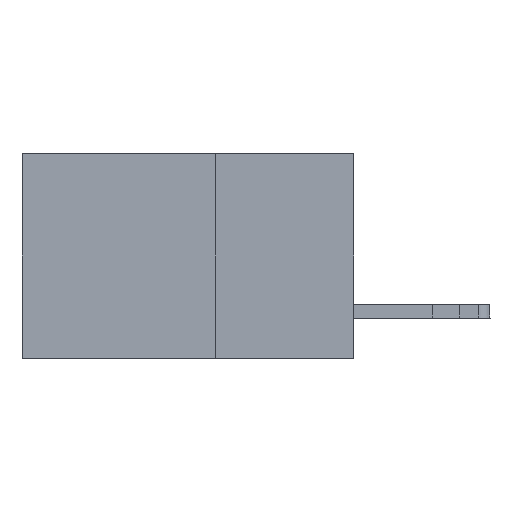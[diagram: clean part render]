
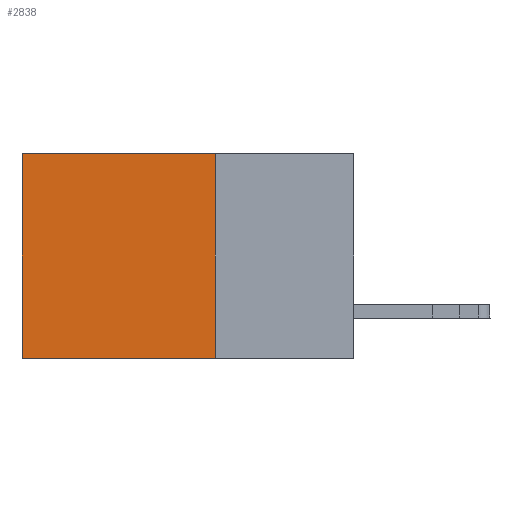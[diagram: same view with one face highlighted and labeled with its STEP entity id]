
A CAD part, left-side view. The second image highlights one B-rep face of the part: STEP entity #2838.
In plain terms, the highlighted planar face has unit normal (-1, 0, 0).
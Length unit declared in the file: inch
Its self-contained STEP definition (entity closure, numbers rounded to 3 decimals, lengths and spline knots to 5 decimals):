
#270 = LINE ( 'NONE', #10448, #17160 ) ;
#1586 = VECTOR ( 'NONE', #26640, 39.37008 ) ;
#2838 = ADVANCED_FACE ( 'NONE', ( #8413 ), #7436, .F. ) ;
#2996 = VECTOR ( 'NONE', #14636, 39.37008 ) ;
#3265 = ORIENTED_EDGE ( 'NONE', *, *, #6133, .T. ) ;
#4250 = AXIS2_PLACEMENT_3D ( 'NONE', #33251, #30945, #9206 ) ;
#6087 = EDGE_CURVE ( 'NONE', #19044, #6957, #270, .T. ) ;
#6133 = EDGE_CURVE ( 'NONE', #6275, #8654, #7215, .T. ) ;
#6275 = VERTEX_POINT ( 'NONE', #22434 ) ;
#6957 = VERTEX_POINT ( 'NONE', #23633 ) ;
#7163 = VECTOR ( 'NONE', #21058, 39.37008 ) ;
#7215 = LINE ( 'NONE', #35376, #1586 ) ;
#7436 = PLANE ( 'NONE',  #4250 ) ;
#7502 = EDGE_CURVE ( 'NONE', #6275, #19044, #20105, .T. ) ;
#8413 = FACE_OUTER_BOUND ( 'NONE', #31206, .T. ) ;
#8654 = VERTEX_POINT ( 'NONE', #25178 ) ;
#9206 = DIRECTION ( 'NONE',  ( 0., 0., -1. ) ) ;
#10448 = CARTESIAN_POINT ( 'NONE',  ( 0.2875, 0.25, -0.37 ) ) ;
#11083 = ORIENTED_EDGE ( 'NONE', *, *, #14413, .T. ) ;
#12601 = CARTESIAN_POINT ( 'NONE',  ( 0.2875, 0.6, 0. ) ) ;
#14413 = EDGE_CURVE ( 'NONE', #8654, #6957, #17717, .T. ) ;
#14636 = DIRECTION ( 'NONE',  ( 0., 0., -1. ) ) ;
#15981 = DIRECTION ( 'NONE',  ( 0., 1., 0. ) ) ;
#17160 = VECTOR ( 'NONE', #15981, 39.37008 ) ;
#17717 = LINE ( 'NONE', #12601, #2996 ) ;
#19044 = VERTEX_POINT ( 'NONE', #26651 ) ;
#20105 = LINE ( 'NONE', #29247, #7163 ) ;
#21058 = DIRECTION ( 'NONE',  ( 0., 0., -1. ) ) ;
#22434 = CARTESIAN_POINT ( 'NONE',  ( 0.2875, 0.25, 0. ) ) ;
#22916 = ORIENTED_EDGE ( 'NONE', *, *, #7502, .F. ) ;
#23633 = CARTESIAN_POINT ( 'NONE',  ( 0.2875, 0.6, -0.37 ) ) ;
#25178 = CARTESIAN_POINT ( 'NONE',  ( 0.2875, 0.6, 0. ) ) ;
#26268 = ORIENTED_EDGE ( 'NONE', *, *, #6087, .F. ) ;
#26640 = DIRECTION ( 'NONE',  ( 0., 1., 0. ) ) ;
#26651 = CARTESIAN_POINT ( 'NONE',  ( 0.2875, 0.25, -0.37 ) ) ;
#29247 = CARTESIAN_POINT ( 'NONE',  ( 0.2875, 0.25, 0. ) ) ;
#30945 = DIRECTION ( 'NONE',  ( 1., 0., 0. ) ) ;
#31206 = EDGE_LOOP ( 'NONE', ( #11083, #26268, #22916, #3265 ) ) ;
#33251 = CARTESIAN_POINT ( 'NONE',  ( 0.2875, 0.25, 0. ) ) ;
#35376 = CARTESIAN_POINT ( 'NONE',  ( 0.2875, 0.25, 0. ) ) ;
